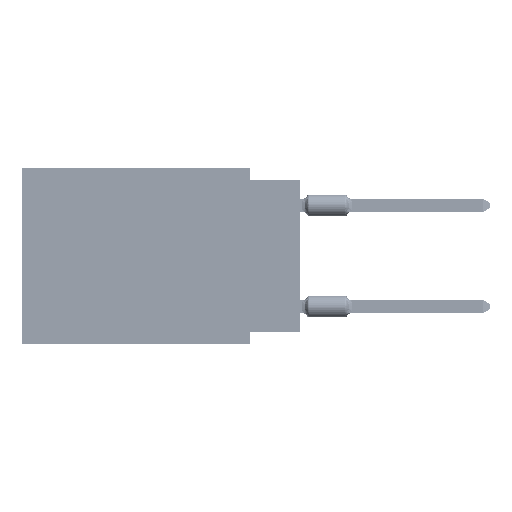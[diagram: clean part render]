
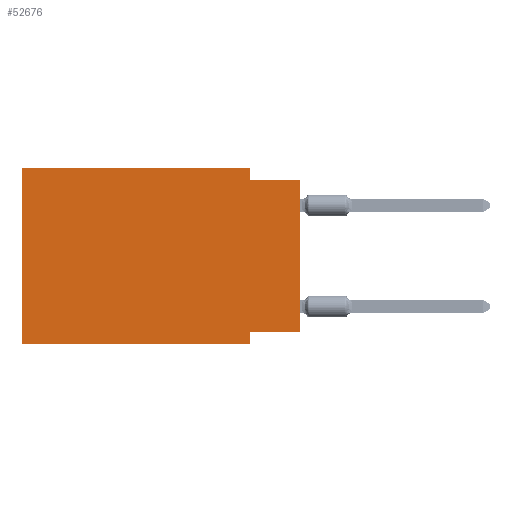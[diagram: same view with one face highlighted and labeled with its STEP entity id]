
A CAD part, left-side view. The second image highlights one B-rep face of the part: STEP entity #52676.
In plain terms, the highlighted planar face has unit normal (-1, 0, 0).
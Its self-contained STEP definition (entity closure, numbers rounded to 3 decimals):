
#2710 = EDGE_LOOP ( 'NONE', ( #4355, #69078, #28944, #58268, #29944, #5098, #22727, #14284 ) ) ;
#2931 = EDGE_CURVE ( 'NONE', #66626, #23504, #56722, .T. ) ;
#3228 = VECTOR ( 'NONE', #28364, 1000. ) ;
#4159 = EDGE_CURVE ( 'NONE', #47503, #30783, #46003, .T. ) ;
#4355 = ORIENTED_EDGE ( 'NONE', *, *, #33006, .T. ) ;
#5098 = ORIENTED_EDGE ( 'NONE', *, *, #63120, .T. ) ;
#5177 = CARTESIAN_POINT ( 'NONE',  ( 0., 0., -8.255 ) ) ;
#5250 = CARTESIAN_POINT ( 'NONE',  ( 0., 13.97, 0. ) ) ;
#5521 = DIRECTION ( 'NONE',  ( 0., -1., 0. ) ) ;
#5614 = CARTESIAN_POINT ( 'NONE',  ( 0., 0., -8.255 ) ) ;
#6237 = LINE ( 'NONE', #37703, #58219 ) ;
#8616 = DIRECTION ( 'NONE',  ( 0., 0., -1. ) ) ;
#10709 = DIRECTION ( 'NONE',  ( 0., 0., -1. ) ) ;
#12605 = DIRECTION ( 'NONE',  ( 1., 0., 0. ) ) ;
#12661 = VECTOR ( 'NONE', #5521, 1000. ) ;
#14284 = ORIENTED_EDGE ( 'NONE', *, *, #2931, .F. ) ;
#17262 = CARTESIAN_POINT ( 'NONE',  ( 0., 13.97, 0. ) ) ;
#17544 = VERTEX_POINT ( 'NONE', #18006 ) ;
#18006 = CARTESIAN_POINT ( 'NONE',  ( 0., 2.54, -8.89 ) ) ;
#20546 = LINE ( 'NONE', #59737, #23455 ) ;
#20989 = VECTOR ( 'NONE', #23017, 1000. ) ;
#22727 = ORIENTED_EDGE ( 'NONE', *, *, #42683, .F. ) ;
#23017 = DIRECTION ( 'NONE',  ( 0., 0., 1. ) ) ;
#23131 = DIRECTION ( 'NONE',  ( 0., -1., 0. ) ) ;
#23455 = VECTOR ( 'NONE', #8616, 1000. ) ;
#23504 = VERTEX_POINT ( 'NONE', #56338 ) ;
#27870 = LINE ( 'NONE', #39809, #20989 ) ;
#28364 = DIRECTION ( 'NONE',  ( 0., 1., 0. ) ) ;
#28834 = DIRECTION ( 'NONE',  ( 0., 0., 1. ) ) ;
#28944 = ORIENTED_EDGE ( 'NONE', *, *, #72291, .F. ) ;
#29944 = ORIENTED_EDGE ( 'NONE', *, *, #4159, .F. ) ;
#30783 = VERTEX_POINT ( 'NONE', #66883 ) ;
#32000 = VECTOR ( 'NONE', #28834, 1000. ) ;
#33006 = EDGE_CURVE ( 'NONE', #66626, #67311, #27870, .T. ) ;
#37587 = VECTOR ( 'NONE', #64992, 1000. ) ;
#37703 = CARTESIAN_POINT ( 'NONE',  ( 0., 2.54, 0. ) ) ;
#39809 = CARTESIAN_POINT ( 'NONE',  ( 0., 0., 0. ) ) ;
#42540 = CARTESIAN_POINT ( 'NONE',  ( 0., 13.97, -8.89 ) ) ;
#42683 = EDGE_CURVE ( 'NONE', #23504, #17544, #20546, .T. ) ;
#45173 = LINE ( 'NONE', #5250, #55536 ) ;
#46003 = LINE ( 'NONE', #17262, #32000 ) ;
#47503 = VERTEX_POINT ( 'NONE', #42540 ) ;
#47686 = FACE_OUTER_BOUND ( 'NONE', #2710, .T. ) ;
#50311 = LINE ( 'NONE', #72332, #12661 ) ;
#51622 = CARTESIAN_POINT ( 'NONE',  ( 0., 2.54, -0.635 ) ) ;
#51860 = AXIS2_PLACEMENT_3D ( 'NONE', #58524, #12605, #64489 ) ;
#52676 = ADVANCED_FACE ( 'NONE', ( #47686 ), #58154, .F. ) ;
#54267 = CARTESIAN_POINT ( 'NONE',  ( 0., 0., -0.635 ) ) ;
#55536 = VECTOR ( 'NONE', #23131, 1000. ) ;
#56338 = CARTESIAN_POINT ( 'NONE',  ( 0., 2.54, -8.255 ) ) ;
#56722 = LINE ( 'NONE', #5614, #3228 ) ;
#58154 = PLANE ( 'NONE',  #51860 ) ;
#58219 = VECTOR ( 'NONE', #10709, 1000. ) ;
#58268 = ORIENTED_EDGE ( 'NONE', *, *, #64007, .F. ) ;
#58524 = CARTESIAN_POINT ( 'NONE',  ( 0., 13.97, 0. ) ) ;
#59131 = VERTEX_POINT ( 'NONE', #51622 ) ;
#59737 = CARTESIAN_POINT ( 'NONE',  ( 0., 2.54, -8.89 ) ) ;
#60054 = VERTEX_POINT ( 'NONE', #61529 ) ;
#61529 = CARTESIAN_POINT ( 'NONE',  ( 0., 2.54, 0. ) ) ;
#63120 = EDGE_CURVE ( 'NONE', #47503, #17544, #50311, .T. ) ;
#63706 = EDGE_CURVE ( 'NONE', #59131, #67311, #69495, .T. ) ;
#64007 = EDGE_CURVE ( 'NONE', #30783, #60054, #45173, .T. ) ;
#64489 = DIRECTION ( 'NONE',  ( 0., 0., -1. ) ) ;
#64992 = DIRECTION ( 'NONE',  ( 0., -1., 0. ) ) ;
#66626 = VERTEX_POINT ( 'NONE', #5177 ) ;
#66883 = CARTESIAN_POINT ( 'NONE',  ( 0., 13.97, 0. ) ) ;
#67311 = VERTEX_POINT ( 'NONE', #54267 ) ;
#69078 = ORIENTED_EDGE ( 'NONE', *, *, #63706, .F. ) ;
#69130 = CARTESIAN_POINT ( 'NONE',  ( 0., 0., -0.635 ) ) ;
#69495 = LINE ( 'NONE', #69130, #37587 ) ;
#72291 = EDGE_CURVE ( 'NONE', #60054, #59131, #6237, .T. ) ;
#72332 = CARTESIAN_POINT ( 'NONE',  ( 0., 13.97, -8.89 ) ) ;
